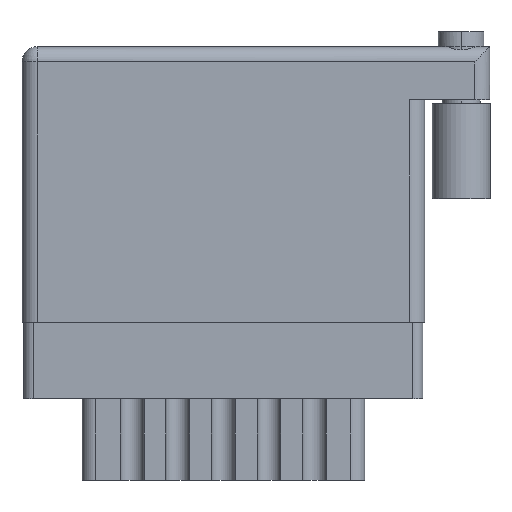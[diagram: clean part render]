
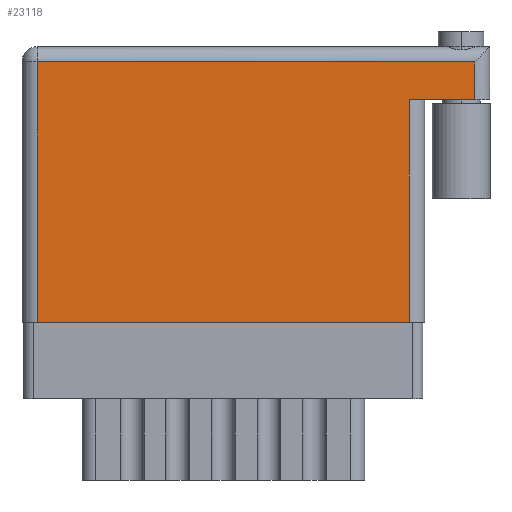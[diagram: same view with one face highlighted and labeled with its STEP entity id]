
A CAD part, front view. The second image highlights one B-rep face of the part: STEP entity #23118.
In plain terms, the highlighted face is planar.
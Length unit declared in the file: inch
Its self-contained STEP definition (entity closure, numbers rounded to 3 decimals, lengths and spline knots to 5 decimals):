
#81 = CARTESIAN_POINT ( 'NONE',  ( 1.489, 0.906, 0. ) ) ;
#397 = DIRECTION ( 'NONE',  ( 0., 1., 0. ) ) ;
#464 = CARTESIAN_POINT ( 'NONE',  ( 0.05, 0., 0. ) ) ;
#840 = AXIS2_PLACEMENT_3D ( 'NONE', #18756, #17048, #8976 ) ;
#995 = FACE_OUTER_BOUND ( 'NONE', #14287, .T. ) ;
#1611 = DIRECTION ( 'NONE',  ( -1., 0., 0. ) ) ;
#4065 = ORIENTED_EDGE ( 'NONE', *, *, #19257, .T. ) ;
#4199 = LINE ( 'NONE', #24283, #7484 ) ;
#4681 = CARTESIAN_POINT ( 'NONE',  ( 0.05, 0.856, 0. ) ) ;
#4984 = EDGE_CURVE ( 'NONE', #20056, #15542, #10145, .T. ) ;
#5162 = LINE ( 'NONE', #19498, #14180 ) ;
#5301 = ORIENTED_EDGE ( 'NONE', *, *, #4984, .T. ) ;
#5680 = VERTEX_POINT ( 'NONE', #17406 ) ;
#7484 = VECTOR ( 'NONE', #12541, 39.37008 ) ;
#8057 = CARTESIAN_POINT ( 'NONE',  ( 1.489, 0.856, 0. ) ) ;
#8433 = EDGE_CURVE ( 'NONE', #12562, #19456, #4199, .T. ) ;
#8750 = DIRECTION ( 'NONE',  ( 1., 0., 0. ) ) ;
#8976 = DIRECTION ( 'NONE',  ( -1., 0., 0. ) ) ;
#9188 = CARTESIAN_POINT ( 'NONE',  ( 1.489, 0.731, 0. ) ) ;
#10145 = LINE ( 'NONE', #81, #23955 ) ;
#10435 = LINE ( 'NONE', #24398, #18131 ) ;
#10659 = DIRECTION ( 'NONE',  ( 0., 1., 0. ) ) ;
#11893 = VECTOR ( 'NONE', #397, 39.37008 ) ;
#12376 = CARTESIAN_POINT ( 'NONE',  ( 1.275, 0.731, 0. ) ) ;
#12541 = DIRECTION ( 'NONE',  ( 0., -1., 0. ) ) ;
#12562 = VERTEX_POINT ( 'NONE', #4681 ) ;
#12955 = EDGE_CURVE ( 'NONE', #20056, #23021, #5162, .T. ) ;
#13600 = LINE ( 'NONE', #25601, #16678 ) ;
#14180 = VECTOR ( 'NONE', #1611, 39.37008 ) ;
#14192 = ORIENTED_EDGE ( 'NONE', *, *, #8433, .T. ) ;
#14287 = EDGE_LOOP ( 'NONE', ( #19164, #22417, #24195, #5301, #4065, #14192 ) ) ;
#15542 = VERTEX_POINT ( 'NONE', #8057 ) ;
#15973 = CARTESIAN_POINT ( 'NONE',  ( 1.275, 0.731, 0. ) ) ;
#16678 = VECTOR ( 'NONE', #21529, 39.37008 ) ;
#17048 = DIRECTION ( 'NONE',  ( 0., 0., -1. ) ) ;
#17387 = EDGE_CURVE ( 'NONE', #19456, #5680, #10435, .T. ) ;
#17406 = CARTESIAN_POINT ( 'NONE',  ( 1.275, 0., 0. ) ) ;
#18131 = VECTOR ( 'NONE', #8750, 39.37008 ) ;
#18756 = CARTESIAN_POINT ( 'NONE',  ( 0., 0.906, 0. ) ) ;
#19164 = ORIENTED_EDGE ( 'NONE', *, *, #17387, .T. ) ;
#19257 = EDGE_CURVE ( 'NONE', #15542, #12562, #13600, .T. ) ;
#19456 = VERTEX_POINT ( 'NONE', #464 ) ;
#19498 = CARTESIAN_POINT ( 'NONE',  ( 1.539, 0.731, 0. ) ) ;
#20056 = VERTEX_POINT ( 'NONE', #9188 ) ;
#20262 = LINE ( 'NONE', #15973, #11893 ) ;
#20333 = EDGE_CURVE ( 'NONE', #5680, #23021, #20262, .T. ) ;
#20705 = PLANE ( 'NONE',  #840 ) ;
#21529 = DIRECTION ( 'NONE',  ( -1., 0., 0. ) ) ;
#22417 = ORIENTED_EDGE ( 'NONE', *, *, #20333, .T. ) ;
#23021 = VERTEX_POINT ( 'NONE', #12376 ) ;
#23118 = ADVANCED_FACE ( 'NONE', ( #995 ), #20705, .F. ) ;
#23955 = VECTOR ( 'NONE', #10659, 39.37008 ) ;
#24195 = ORIENTED_EDGE ( 'NONE', *, *, #12955, .F. ) ;
#24283 = CARTESIAN_POINT ( 'NONE',  ( 0.05, 0., 0. ) ) ;
#24398 = CARTESIAN_POINT ( 'NONE',  ( 0., 0., 0. ) ) ;
#25601 = CARTESIAN_POINT ( 'NONE',  ( 0., 0.856, 0. ) ) ;
